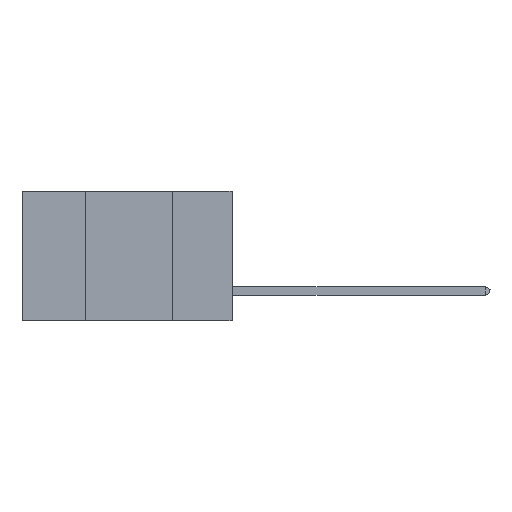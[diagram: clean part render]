
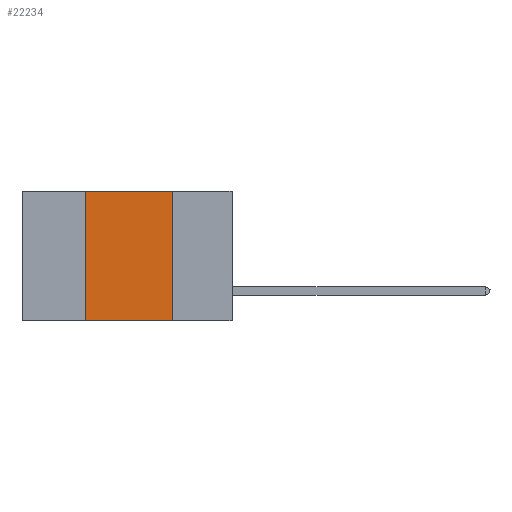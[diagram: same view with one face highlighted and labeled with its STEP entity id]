
A CAD part, left-side view. The second image highlights one B-rep face of the part: STEP entity #22234.
In plain terms, the highlighted planar face has unit normal (-1, 0, 0).
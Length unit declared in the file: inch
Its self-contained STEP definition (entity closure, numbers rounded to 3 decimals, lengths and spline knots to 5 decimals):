
#154 = DIRECTION ( 'NONE',  ( 0., -1., 0. ) ) ;
#608 = LINE ( 'NONE', #6516, #33776 ) ;
#1843 = PLANE ( 'NONE',  #37723 ) ;
#5202 = CARTESIAN_POINT ( 'NONE',  ( 0., 0.6, 0. ) ) ;
#6381 = DIRECTION ( 'NONE',  ( 0., 0., 1. ) ) ;
#6516 = CARTESIAN_POINT ( 'NONE',  ( 0., 0.42, 0. ) ) ;
#8513 = VECTOR ( 'NONE', #34054, 39.37008 ) ;
#9268 = ORIENTED_EDGE ( 'NONE', *, *, #26575, .F. ) ;
#9485 = VERTEX_POINT ( 'NONE', #31939 ) ;
#9926 = VERTEX_POINT ( 'NONE', #17897 ) ;
#10525 = EDGE_CURVE ( 'NONE', #27959, #9926, #18112, .T. ) ;
#11053 = ORIENTED_EDGE ( 'NONE', *, *, #10525, .T. ) ;
#11236 = DIRECTION ( 'NONE',  ( 0., 0., -1. ) ) ;
#14755 = VERTEX_POINT ( 'NONE', #26110 ) ;
#15634 = LINE ( 'NONE', #19208, #40314 ) ;
#15856 = EDGE_LOOP ( 'NONE', ( #41202, #9268, #29152, #11053 ) ) ;
#16818 = EDGE_CURVE ( 'NONE', #14755, #9926, #17506, .T. ) ;
#16979 = FACE_OUTER_BOUND ( 'NONE', #15856, .T. ) ;
#17506 = LINE ( 'NONE', #24055, #8513 ) ;
#17897 = CARTESIAN_POINT ( 'NONE',  ( 0., 0.17, -0.37 ) ) ;
#17963 = CARTESIAN_POINT ( 'NONE',  ( 0., 0.42, -0.37 ) ) ;
#18112 = LINE ( 'NONE', #23178, #20135 ) ;
#19208 = CARTESIAN_POINT ( 'NONE',  ( 0., 0.6, 0. ) ) ;
#20135 = VECTOR ( 'NONE', #36141, 39.37008 ) ;
#22234 = ADVANCED_FACE ( 'NONE', ( #16979 ), #1843, .F. ) ;
#23178 = CARTESIAN_POINT ( 'NONE',  ( 0., 0.6, -0.37 ) ) ;
#24055 = CARTESIAN_POINT ( 'NONE',  ( 0., 0.17, 0. ) ) ;
#26110 = CARTESIAN_POINT ( 'NONE',  ( 0., 0.17, 0. ) ) ;
#26575 = EDGE_CURVE ( 'NONE', #9485, #14755, #15634, .T. ) ;
#27959 = VERTEX_POINT ( 'NONE', #17963 ) ;
#29152 = ORIENTED_EDGE ( 'NONE', *, *, #29463, .F. ) ;
#29463 = EDGE_CURVE ( 'NONE', #27959, #9485, #608, .T. ) ;
#31939 = CARTESIAN_POINT ( 'NONE',  ( 0., 0.42, 0. ) ) ;
#33776 = VECTOR ( 'NONE', #6381, 39.37008 ) ;
#34054 = DIRECTION ( 'NONE',  ( 0., 0., -1. ) ) ;
#36141 = DIRECTION ( 'NONE',  ( 0., -1., 0. ) ) ;
#37723 = AXIS2_PLACEMENT_3D ( 'NONE', #5202, #40479, #11236 ) ;
#40314 = VECTOR ( 'NONE', #154, 39.37008 ) ;
#40479 = DIRECTION ( 'NONE',  ( 1., 0., 0. ) ) ;
#41202 = ORIENTED_EDGE ( 'NONE', *, *, #16818, .F. ) ;
